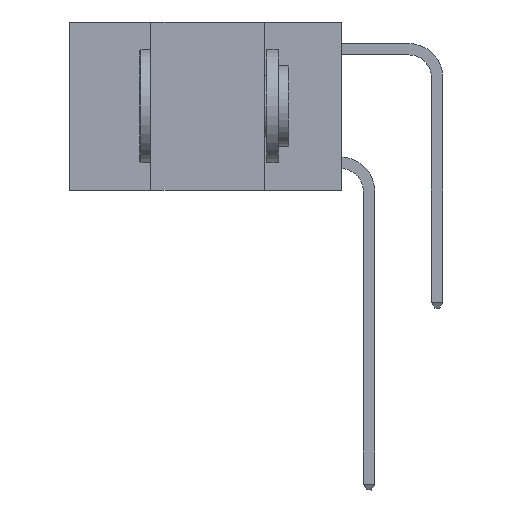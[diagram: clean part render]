
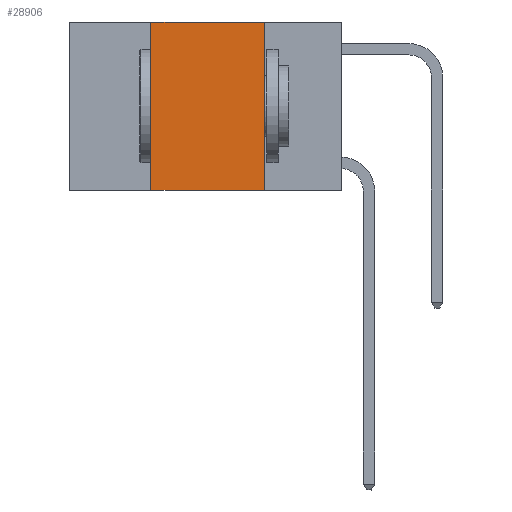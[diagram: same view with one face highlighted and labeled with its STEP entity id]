
A CAD part, left-side view. The second image highlights one B-rep face of the part: STEP entity #28906.
In plain terms, the highlighted planar face has unit normal (-1, 0, 0).
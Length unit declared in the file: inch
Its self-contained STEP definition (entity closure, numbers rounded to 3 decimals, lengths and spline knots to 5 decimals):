
#1587 = VECTOR ( 'NONE', #23279, 39.37008 ) ;
#2590 = VERTEX_POINT ( 'NONE', #17725 ) ;
#5305 = CARTESIAN_POINT ( 'NONE',  ( 0., 0.6, -0.37 ) ) ;
#6226 = EDGE_CURVE ( 'NONE', #30529, #17350, #11641, .T. ) ;
#6278 = LINE ( 'NONE', #11433, #19702 ) ;
#7424 = EDGE_CURVE ( 'NONE', #24642, #17350, #10448, .T. ) ;
#7736 = ORIENTED_EDGE ( 'NONE', *, *, #18828, .F. ) ;
#8105 = DIRECTION ( 'NONE',  ( 0., -1., 0. ) ) ;
#8283 = ORIENTED_EDGE ( 'NONE', *, *, #26517, .F. ) ;
#9956 = VECTOR ( 'NONE', #8105, 39.37008 ) ;
#10448 = LINE ( 'NONE', #5305, #9956 ) ;
#11433 = CARTESIAN_POINT ( 'NONE',  ( 0., 0.6, 0. ) ) ;
#11641 = LINE ( 'NONE', #30017, #25244 ) ;
#13083 = LINE ( 'NONE', #18424, #1587 ) ;
#14686 = AXIS2_PLACEMENT_3D ( 'NONE', #14724, #24291, #25069 ) ;
#14694 = ORIENTED_EDGE ( 'NONE', *, *, #7424, .T. ) ;
#14724 = CARTESIAN_POINT ( 'NONE',  ( 0., 0.6, 0. ) ) ;
#15818 = DIRECTION ( 'NONE',  ( 0., -1., 0. ) ) ;
#16467 = EDGE_LOOP ( 'NONE', ( #17629, #7736, #8283, #14694 ) ) ;
#17350 = VERTEX_POINT ( 'NONE', #22975 ) ;
#17629 = ORIENTED_EDGE ( 'NONE', *, *, #6226, .F. ) ;
#17725 = CARTESIAN_POINT ( 'NONE',  ( 0., 0.42, 0. ) ) ;
#17861 = PLANE ( 'NONE',  #14686 ) ;
#18424 = CARTESIAN_POINT ( 'NONE',  ( 0., 0.42, 0. ) ) ;
#18828 = EDGE_CURVE ( 'NONE', #2590, #30529, #6278, .T. ) ;
#19702 = VECTOR ( 'NONE', #15818, 39.37008 ) ;
#21752 = CARTESIAN_POINT ( 'NONE',  ( 0., 0.17, 0. ) ) ;
#22560 = FACE_OUTER_BOUND ( 'NONE', #16467, .T. ) ;
#22975 = CARTESIAN_POINT ( 'NONE',  ( 0., 0.17, -0.37 ) ) ;
#23096 = DIRECTION ( 'NONE',  ( 0., 0., -1. ) ) ;
#23279 = DIRECTION ( 'NONE',  ( 0., 0., 1. ) ) ;
#24291 = DIRECTION ( 'NONE',  ( 1., 0., 0. ) ) ;
#24642 = VERTEX_POINT ( 'NONE', #25043 ) ;
#25043 = CARTESIAN_POINT ( 'NONE',  ( 0., 0.42, -0.37 ) ) ;
#25069 = DIRECTION ( 'NONE',  ( 0., 0., -1. ) ) ;
#25244 = VECTOR ( 'NONE', #23096, 39.37008 ) ;
#26517 = EDGE_CURVE ( 'NONE', #24642, #2590, #13083, .T. ) ;
#28906 = ADVANCED_FACE ( 'NONE', ( #22560 ), #17861, .F. ) ;
#30017 = CARTESIAN_POINT ( 'NONE',  ( 0., 0.17, 0. ) ) ;
#30529 = VERTEX_POINT ( 'NONE', #21752 ) ;
